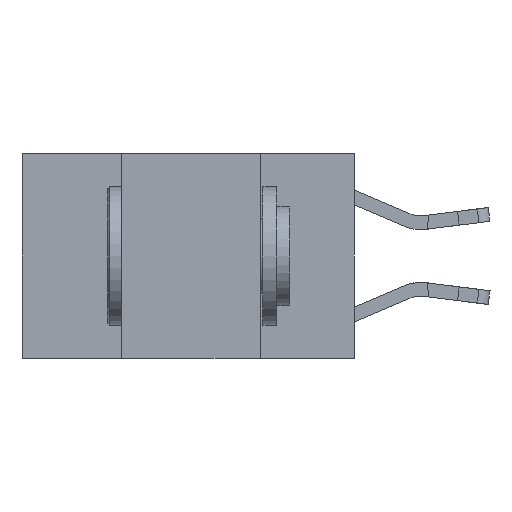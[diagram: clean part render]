
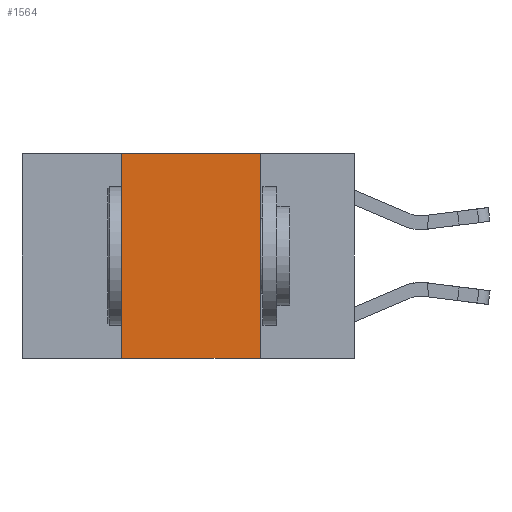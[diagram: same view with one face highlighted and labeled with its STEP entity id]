
A CAD part, left-side view. The second image highlights one B-rep face of the part: STEP entity #1564.
In plain terms, the highlighted planar face has unit normal (-1, 0, 0).
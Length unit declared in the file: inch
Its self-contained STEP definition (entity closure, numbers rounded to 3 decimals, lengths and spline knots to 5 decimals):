
#650 = DIRECTION ( 'NONE',  ( 0., -1., 0. ) ) ;
#1564 = ADVANCED_FACE ( 'NONE', ( #9731 ), #23147, .F. ) ;
#2057 = CARTESIAN_POINT ( 'NONE',  ( 0., 0.6, -0.37 ) ) ;
#2351 = VECTOR ( 'NONE', #5637, 39.37008 ) ;
#3878 = EDGE_LOOP ( 'NONE', ( #13591, #16160, #9144, #14564 ) ) ;
#5197 = VECTOR ( 'NONE', #650, 39.37008 ) ;
#5637 = DIRECTION ( 'NONE',  ( 0., 0., 1. ) ) ;
#6229 = VERTEX_POINT ( 'NONE', #10145 ) ;
#7907 = LINE ( 'NONE', #13818, #2351 ) ;
#9144 = ORIENTED_EDGE ( 'NONE', *, *, #23489, .F. ) ;
#9683 = CARTESIAN_POINT ( 'NONE',  ( 0., 0.17, -0.37 ) ) ;
#9731 = FACE_OUTER_BOUND ( 'NONE', #3878, .T. ) ;
#9873 = CARTESIAN_POINT ( 'NONE',  ( 0., 0.17, 0. ) ) ;
#10145 = CARTESIAN_POINT ( 'NONE',  ( 0., 0.42, 0. ) ) ;
#10996 = CARTESIAN_POINT ( 'NONE',  ( 0., 0.6, 0. ) ) ;
#11043 = VERTEX_POINT ( 'NONE', #11963 ) ;
#11963 = CARTESIAN_POINT ( 'NONE',  ( 0., 0.17, 0. ) ) ;
#12444 = LINE ( 'NONE', #9873, #22583 ) ;
#13591 = ORIENTED_EDGE ( 'NONE', *, *, #22154, .F. ) ;
#13818 = CARTESIAN_POINT ( 'NONE',  ( 0., 0.42, 0. ) ) ;
#14564 = ORIENTED_EDGE ( 'NONE', *, *, #20244, .T. ) ;
#16160 = ORIENTED_EDGE ( 'NONE', *, *, #19086, .F. ) ;
#16390 = AXIS2_PLACEMENT_3D ( 'NONE', #23378, #22951, #22918 ) ;
#18757 = VERTEX_POINT ( 'NONE', #24299 ) ;
#19086 = EDGE_CURVE ( 'NONE', #6229, #11043, #21479, .T. ) ;
#19837 = LINE ( 'NONE', #2057, #24564 ) ;
#20244 = EDGE_CURVE ( 'NONE', #18757, #20720, #19837, .T. ) ;
#20525 = DIRECTION ( 'NONE',  ( 0., -1., 0. ) ) ;
#20720 = VERTEX_POINT ( 'NONE', #9683 ) ;
#21479 = LINE ( 'NONE', #10996, #5197 ) ;
#22154 = EDGE_CURVE ( 'NONE', #11043, #20720, #12444, .T. ) ;
#22583 = VECTOR ( 'NONE', #26067, 39.37008 ) ;
#22918 = DIRECTION ( 'NONE',  ( 0., 0., -1. ) ) ;
#22951 = DIRECTION ( 'NONE',  ( 1., 0., 0. ) ) ;
#23147 = PLANE ( 'NONE',  #16390 ) ;
#23378 = CARTESIAN_POINT ( 'NONE',  ( 0., 0.6, 0. ) ) ;
#23489 = EDGE_CURVE ( 'NONE', #18757, #6229, #7907, .T. ) ;
#24299 = CARTESIAN_POINT ( 'NONE',  ( 0., 0.42, -0.37 ) ) ;
#24564 = VECTOR ( 'NONE', #20525, 39.37008 ) ;
#26067 = DIRECTION ( 'NONE',  ( 0., 0., -1. ) ) ;
